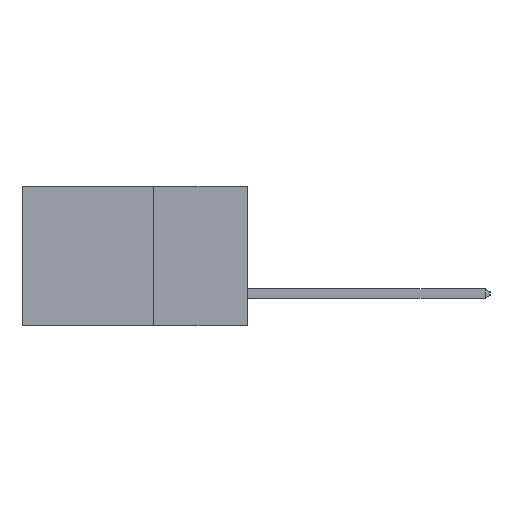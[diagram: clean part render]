
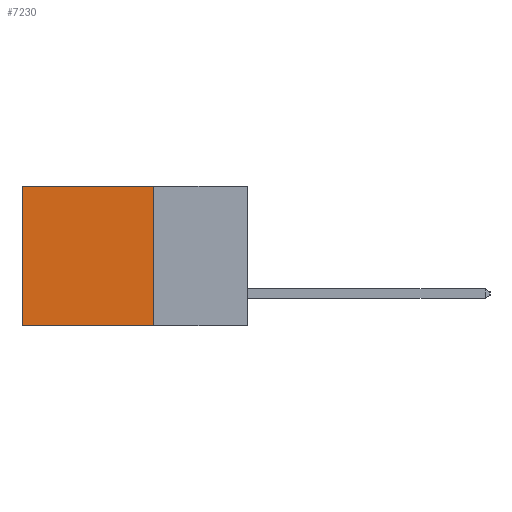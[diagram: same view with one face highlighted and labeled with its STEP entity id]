
A CAD part, left-side view. The second image highlights one B-rep face of the part: STEP entity #7230.
In plain terms, the highlighted planar face has unit normal (-1, 0, 0).
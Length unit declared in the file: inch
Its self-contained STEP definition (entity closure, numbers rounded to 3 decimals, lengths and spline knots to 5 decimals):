
#383 = CARTESIAN_POINT ( 'NONE',  ( 0.2615, 0.25, -0.37 ) ) ;
#508 = DIRECTION ( 'NONE',  ( 0., 1., 0. ) ) ;
#709 = CARTESIAN_POINT ( 'NONE',  ( 0.2615, 0.6, 0. ) ) ;
#886 = EDGE_CURVE ( 'NONE', #6918, #9741, #7740, .T. ) ;
#894 = DIRECTION ( 'NONE',  ( 0., 1., 0. ) ) ;
#1226 = ORIENTED_EDGE ( 'NONE', *, *, #886, .T. ) ;
#1401 = CARTESIAN_POINT ( 'NONE',  ( 0.2615, 0.25, 0. ) ) ;
#2533 = ORIENTED_EDGE ( 'NONE', *, *, #3957, .F. ) ;
#2622 = ORIENTED_EDGE ( 'NONE', *, *, #10209, .F. ) ;
#2748 = ORIENTED_EDGE ( 'NONE', *, *, #3663, .T. ) ;
#3079 = VECTOR ( 'NONE', #894, 39.37008 ) ;
#3172 = AXIS2_PLACEMENT_3D ( 'NONE', #3712, #9299, #4544 ) ;
#3663 = EDGE_CURVE ( 'NONE', #5629, #6918, #9235, .T. ) ;
#3712 = CARTESIAN_POINT ( 'NONE',  ( 0.2615, 0.25, -0.37 ) ) ;
#3797 = CARTESIAN_POINT ( 'NONE',  ( 0.2615, 0.25, -0.37 ) ) ;
#3957 = EDGE_CURVE ( 'NONE', #9286, #9741, #6962, .T. ) ;
#4544 = DIRECTION ( 'NONE',  ( 0., 0., -1. ) ) ;
#4982 = FACE_OUTER_BOUND ( 'NONE', #9205, .T. ) ;
#5215 = LINE ( 'NONE', #383, #5480 ) ;
#5332 = VECTOR ( 'NONE', #9677, 39.37008 ) ;
#5480 = VECTOR ( 'NONE', #6332, 39.37008 ) ;
#5629 = VERTEX_POINT ( 'NONE', #5880 ) ;
#5880 = CARTESIAN_POINT ( 'NONE',  ( 0.2615, 0.25, 0. ) ) ;
#5979 = CARTESIAN_POINT ( 'NONE',  ( 0.2615, 0.25, -0.37 ) ) ;
#6332 = DIRECTION ( 'NONE',  ( 0., 0., -1. ) ) ;
#6918 = VERTEX_POINT ( 'NONE', #709 ) ;
#6962 = LINE ( 'NONE', #5979, #3079 ) ;
#7207 = VECTOR ( 'NONE', #508, 39.37008 ) ;
#7230 = ADVANCED_FACE ( 'NONE', ( #4982 ), #7788, .F. ) ;
#7740 = LINE ( 'NONE', #9844, #5332 ) ;
#7788 = PLANE ( 'NONE',  #3172 ) ;
#9205 = EDGE_LOOP ( 'NONE', ( #1226, #2533, #2622, #2748 ) ) ;
#9235 = LINE ( 'NONE', #1401, #7207 ) ;
#9286 = VERTEX_POINT ( 'NONE', #3797 ) ;
#9299 = DIRECTION ( 'NONE',  ( 1., 0., 0. ) ) ;
#9677 = DIRECTION ( 'NONE',  ( 0., 0., -1. ) ) ;
#9741 = VERTEX_POINT ( 'NONE', #10274 ) ;
#9844 = CARTESIAN_POINT ( 'NONE',  ( 0.2615, 0.6, -0.37 ) ) ;
#10209 = EDGE_CURVE ( 'NONE', #5629, #9286, #5215, .T. ) ;
#10274 = CARTESIAN_POINT ( 'NONE',  ( 0.2615, 0.6, -0.37 ) ) ;
